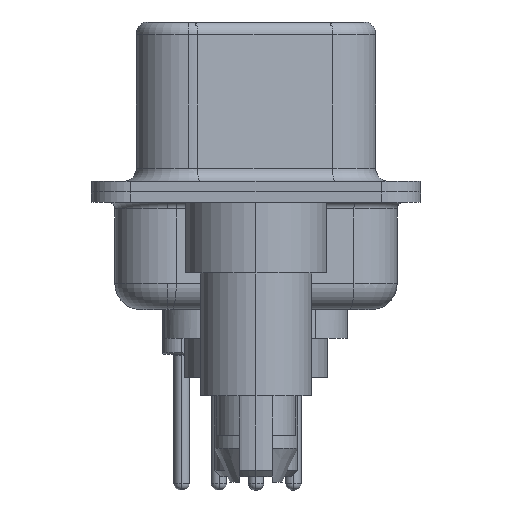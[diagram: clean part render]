
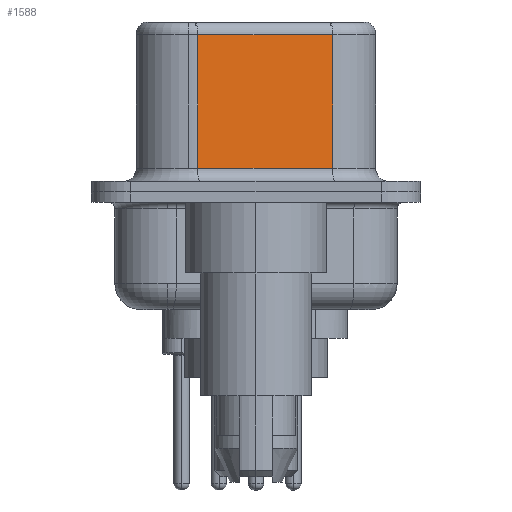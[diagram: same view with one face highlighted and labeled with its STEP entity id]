
A CAD part, left-side view. The second image highlights one B-rep face of the part: STEP entity #1588.
In plain terms, the highlighted planar face has unit normal (-0.985, -0.174, 0).
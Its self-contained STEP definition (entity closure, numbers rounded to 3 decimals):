
#845 = LINE ( 'NONE', #24961, #11644 ) ;
#874 = ORIENTED_EDGE ( 'NONE', *, *, #8106, .T. ) ;
#1588 = ADVANCED_FACE ( 'NONE', ( #6192 ), #15348, .F. ) ;
#2831 = DIRECTION ( 'NONE',  ( -0.174, 0.985, 0. ) ) ;
#2832 = VERTEX_POINT ( 'NONE', #17038 ) ;
#3257 = CARTESIAN_POINT ( 'NONE',  ( 4.58, -2.927, 6.02 ) ) ;
#4380 = VERTEX_POINT ( 'NONE', #22298 ) ;
#6192 = FACE_OUTER_BOUND ( 'NONE', #12177, .T. ) ;
#6649 = ORIENTED_EDGE ( 'NONE', *, *, #17901, .T. ) ;
#7420 = VECTOR ( 'NONE', #18416, 1000. ) ;
#8106 = EDGE_CURVE ( 'NONE', #4380, #2832, #19131, .T. ) ;
#9330 = VERTEX_POINT ( 'NONE', #3257 ) ;
#9424 = CARTESIAN_POINT ( 'NONE',  ( 4.58, -2.927, 6.52 ) ) ;
#9811 = CARTESIAN_POINT ( 'NONE',  ( 4.58, -2.927, 0.9 ) ) ;
#10224 = DIRECTION ( 'NONE',  ( 0.174, -0.985, 0. ) ) ;
#11644 = VECTOR ( 'NONE', #14348, 1000. ) ;
#12177 = EDGE_LOOP ( 'NONE', ( #12873, #6649, #874, #25636 ) ) ;
#12857 = LINE ( 'NONE', #23054, #24876 ) ;
#12873 = ORIENTED_EDGE ( 'NONE', *, *, #16580, .F. ) ;
#14325 = CARTESIAN_POINT ( 'NONE',  ( 3.67, 2.233, 6.52 ) ) ;
#14348 = DIRECTION ( 'NONE',  ( -0.174, 0.985, 0. ) ) ;
#15131 = EDGE_CURVE ( 'NONE', #2832, #18484, #12857, .T. ) ;
#15348 = PLANE ( 'NONE',  #25307 ) ;
#16580 = EDGE_CURVE ( 'NONE', #9330, #18484, #18215, .T. ) ;
#17038 = CARTESIAN_POINT ( 'NONE',  ( 3.67, 2.233, 0.9 ) ) ;
#17901 = EDGE_CURVE ( 'NONE', #9330, #4380, #845, .T. ) ;
#18215 = LINE ( 'NONE', #9424, #7420 ) ;
#18416 = DIRECTION ( 'NONE',  ( 0., 0., -1. ) ) ;
#18484 = VERTEX_POINT ( 'NONE', #9811 ) ;
#19131 = LINE ( 'NONE', #14325, #24062 ) ;
#21812 = CARTESIAN_POINT ( 'NONE',  ( 4.58, -2.927, 6.52 ) ) ;
#22082 = DIRECTION ( 'NONE',  ( 0.985, 0.174, 0. ) ) ;
#22298 = CARTESIAN_POINT ( 'NONE',  ( 3.67, 2.233, 6.02 ) ) ;
#23054 = CARTESIAN_POINT ( 'NONE',  ( 4.58, -2.927, 0.9 ) ) ;
#24062 = VECTOR ( 'NONE', #27016, 1000. ) ;
#24876 = VECTOR ( 'NONE', #10224, 1000. ) ;
#24961 = CARTESIAN_POINT ( 'NONE',  ( 4.58, -2.927, 6.02 ) ) ;
#25307 = AXIS2_PLACEMENT_3D ( 'NONE', #21812, #22082, #2831 ) ;
#25636 = ORIENTED_EDGE ( 'NONE', *, *, #15131, .T. ) ;
#27016 = DIRECTION ( 'NONE',  ( 0., 0., -1. ) ) ;
